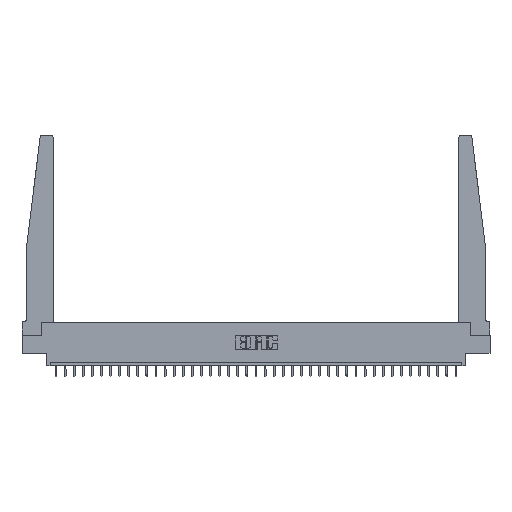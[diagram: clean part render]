
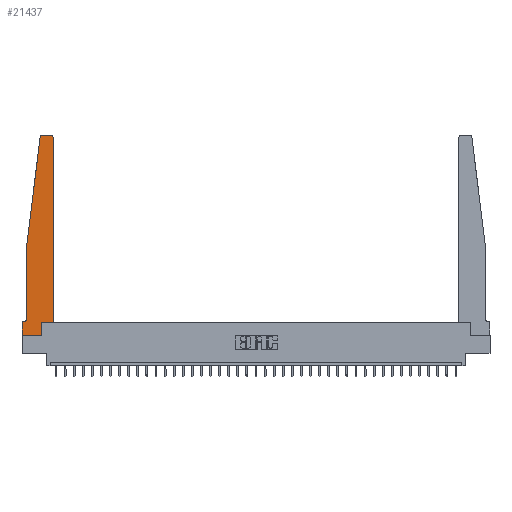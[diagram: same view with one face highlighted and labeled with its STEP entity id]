
A CAD part, top view. The second image highlights one B-rep face of the part: STEP entity #21437.
In plain terms, the highlighted planar face has unit normal (0, 0, 1).
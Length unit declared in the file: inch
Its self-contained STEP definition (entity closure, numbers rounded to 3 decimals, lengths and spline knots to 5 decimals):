
#78 = CARTESIAN_POINT ( 'NONE',  ( 0.015, 0.2375, 0.37 ) ) ;
#436 = CARTESIAN_POINT ( 'NONE',  ( 0., 0., 0.37 ) ) ;
#1081 = ORIENTED_EDGE ( 'NONE', *, *, #4601, .T. ) ;
#1486 = DIRECTION ( 'NONE',  ( 0., -1., 0. ) ) ;
#1632 = CARTESIAN_POINT ( 'NONE',  ( 0., 0., 0.37 ) ) ;
#1698 = CARTESIAN_POINT ( 'NONE',  ( 0.2605, 0., 0.37 ) ) ;
#1719 = VECTOR ( 'NONE', #17301, 39.37008 ) ;
#1844 = CARTESIAN_POINT ( 'NONE',  ( 0.425, 0.18, 0.37 ) ) ;
#1995 = EDGE_CURVE ( 'NONE', #14347, #32443, #30287, .T. ) ;
#2155 = CARTESIAN_POINT ( 'NONE',  ( 0., 0., 0.37 ) ) ;
#2578 = DIRECTION ( 'NONE',  ( 1., 0., 0. ) ) ;
#2686 = EDGE_LOOP ( 'NONE', ( #14215, #1081, #5390, #25383, #31461, #9078, #31612, #27559, #22844, #9405, #11229, #5783 ) ) ;
#2786 = EDGE_CURVE ( 'NONE', #32053, #6396, #11016, .T. ) ;
#2797 = VERTEX_POINT ( 'NONE', #1698 ) ;
#3296 = VERTEX_POINT ( 'NONE', #436 ) ;
#4121 = EDGE_CURVE ( 'NONE', #10559, #21820, #5808, .T. ) ;
#4601 = EDGE_CURVE ( 'NONE', #23123, #32053, #27783, .T. ) ;
#4746 = CARTESIAN_POINT ( 'NONE',  ( 0.425, 0.18, 0.37 ) ) ;
#5390 = ORIENTED_EDGE ( 'NONE', *, *, #2786, .T. ) ;
#5399 = DIRECTION ( 'NONE',  ( 0., 0., 1. ) ) ;
#5516 = CIRCLE ( 'NONE', #15982, 0.05 ) ;
#5783 = ORIENTED_EDGE ( 'NONE', *, *, #4121, .T. ) ;
#5808 = CIRCLE ( 'NONE', #29181, 0.03 ) ;
#6149 = CARTESIAN_POINT ( 'NONE',  ( 0.2605, 0.18, 0.37 ) ) ;
#6396 = VERTEX_POINT ( 'NONE', #20817 ) ;
#6866 = DIRECTION ( 'NONE',  ( 0., -1., 0. ) ) ;
#7437 = EDGE_CURVE ( 'NONE', #2797, #14347, #8352, .T. ) ;
#7590 = DIRECTION ( 'NONE',  ( 1., 0., 0. ) ) ;
#7659 = VERTEX_POINT ( 'NONE', #28239 ) ;
#7867 = EDGE_CURVE ( 'NONE', #32443, #10559, #13844, .T. ) ;
#8148 = CARTESIAN_POINT ( 'NONE',  ( 0.425, 2.72, 0.37 ) ) ;
#8352 = LINE ( 'NONE', #6149, #1719 ) ;
#8532 = EDGE_CURVE ( 'NONE', #21820, #23123, #30784, .T. ) ;
#8833 = VECTOR ( 'NONE', #8940, 39.37008 ) ;
#8940 = DIRECTION ( 'NONE',  ( -1., 0., 0. ) ) ;
#9078 = ORIENTED_EDGE ( 'NONE', *, *, #15587, .T. ) ;
#9405 = ORIENTED_EDGE ( 'NONE', *, *, #1995, .T. ) ;
#10381 = DIRECTION ( 'NONE',  ( 1., 0., 0. ) ) ;
#10559 = VERTEX_POINT ( 'NONE', #8148 ) ;
#10767 = VECTOR ( 'NONE', #26621, 39.37008 ) ;
#11016 = LINE ( 'NONE', #21911, #14957 ) ;
#11229 = ORIENTED_EDGE ( 'NONE', *, *, #7867, .T. ) ;
#11241 = DIRECTION ( 'NONE',  ( 1., 0., 0. ) ) ;
#11785 = DIRECTION ( 'NONE',  ( 0., 1., 0. ) ) ;
#12787 = PLANE ( 'NONE',  #24718 ) ;
#12901 = DIRECTION ( 'NONE',  ( 0., 0., 1. ) ) ;
#13844 = LINE ( 'NONE', #4746, #32254 ) ;
#14215 = ORIENTED_EDGE ( 'NONE', *, *, #8532, .T. ) ;
#14238 = DIRECTION ( 'NONE',  ( 1., 0., 0. ) ) ;
#14347 = VERTEX_POINT ( 'NONE', #21317 ) ;
#14620 = DIRECTION ( 'NONE',  ( -0.122, -0.992, 0. ) ) ;
#14957 = VECTOR ( 'NONE', #14620, 39.37008 ) ;
#15138 = CARTESIAN_POINT ( 'NONE',  ( 0.27653, 2.75, 0.37 ) ) ;
#15587 = EDGE_CURVE ( 'NONE', #7659, #31691, #28891, .T. ) ;
#15982 = AXIS2_PLACEMENT_3D ( 'NONE', #78, #24930, #17506 ) ;
#16224 = CARTESIAN_POINT ( 'NONE',  ( 0.395, 2.72, 0.37 ) ) ;
#16771 = CARTESIAN_POINT ( 'NONE',  ( 0.065, 1.25, 0.37 ) ) ;
#17044 = CARTESIAN_POINT ( 'NONE',  ( 0.065, 0.2375, 0.37 ) ) ;
#17201 = CARTESIAN_POINT ( 'NONE',  ( 0.24675, 2.72367, 0.37 ) ) ;
#17301 = DIRECTION ( 'NONE',  ( 0., 1., 0. ) ) ;
#17506 = DIRECTION ( 'NONE',  ( -1., 0., 0. ) ) ;
#19247 = LINE ( 'NONE', #2155, #21205 ) ;
#19880 = VERTEX_POINT ( 'NONE', #17044 ) ;
#20494 = CARTESIAN_POINT ( 'NONE',  ( 0.27653, 2.72, 0.37 ) ) ;
#20817 = CARTESIAN_POINT ( 'NONE',  ( 0.065, 1.25, 0.37 ) ) ;
#21205 = VECTOR ( 'NONE', #2578, 39.37008 ) ;
#21317 = CARTESIAN_POINT ( 'NONE',  ( 0.2605, 0.18, 0.37 ) ) ;
#21415 = CARTESIAN_POINT ( 'NONE',  ( 0.065, 0.1875, 0.37 ) ) ;
#21437 = ADVANCED_FACE ( 'NONE', ( #24043 ), #12787, .T. ) ;
#21820 = VERTEX_POINT ( 'NONE', #31414 ) ;
#21911 = CARTESIAN_POINT ( 'NONE',  ( 0.065, 1.25, 0.37 ) ) ;
#22844 = ORIENTED_EDGE ( 'NONE', *, *, #7437, .T. ) ;
#23088 = LINE ( 'NONE', #1632, #30123 ) ;
#23123 = VERTEX_POINT ( 'NONE', #15138 ) ;
#23212 = EDGE_CURVE ( 'NONE', #19880, #7659, #5516, .T. ) ;
#23755 = DIRECTION ( 'NONE',  ( 0., 0., 1. ) ) ;
#24043 = FACE_OUTER_BOUND ( 'NONE', #2686, .T. ) ;
#24074 = CARTESIAN_POINT ( 'NONE',  ( 0.425, 0.18, 0.37 ) ) ;
#24140 = CARTESIAN_POINT ( 'NONE',  ( 0.25, 2.75, 0.37 ) ) ;
#24223 = VECTOR ( 'NONE', #1486, 39.37008 ) ;
#24374 = EDGE_CURVE ( 'NONE', #3296, #2797, #19247, .T. ) ;
#24579 = LINE ( 'NONE', #16771, #24223 ) ;
#24718 = AXIS2_PLACEMENT_3D ( 'NONE', #27707, #12901, #10381 ) ;
#24930 = DIRECTION ( 'NONE',  ( 0., 0., -1. ) ) ;
#24989 = CARTESIAN_POINT ( 'NONE',  ( 0., 0.1875, 0.37 ) ) ;
#25383 = ORIENTED_EDGE ( 'NONE', *, *, #29550, .T. ) ;
#25432 = AXIS2_PLACEMENT_3D ( 'NONE', #20494, #5399, #7590 ) ;
#26621 = DIRECTION ( 'NONE',  ( -1., 0., 0. ) ) ;
#27559 = ORIENTED_EDGE ( 'NONE', *, *, #24374, .T. ) ;
#27707 = CARTESIAN_POINT ( 'NONE',  ( 0., 0.1875, 0.37 ) ) ;
#27783 = CIRCLE ( 'NONE', #25432, 0.03 ) ;
#27932 = VECTOR ( 'NONE', #14238, 39.37008 ) ;
#28239 = CARTESIAN_POINT ( 'NONE',  ( 0.015, 0.1875, 0.37 ) ) ;
#28240 = EDGE_CURVE ( 'NONE', #31691, #3296, #23088, .T. ) ;
#28891 = LINE ( 'NONE', #21415, #8833 ) ;
#29181 = AXIS2_PLACEMENT_3D ( 'NONE', #16224, #23755, #11241 ) ;
#29550 = EDGE_CURVE ( 'NONE', #6396, #19880, #24579, .T. ) ;
#30123 = VECTOR ( 'NONE', #6866, 39.37008 ) ;
#30287 = LINE ( 'NONE', #1844, #27932 ) ;
#30784 = LINE ( 'NONE', #24140, #10767 ) ;
#31414 = CARTESIAN_POINT ( 'NONE',  ( 0.395, 2.75, 0.37 ) ) ;
#31461 = ORIENTED_EDGE ( 'NONE', *, *, #23212, .T. ) ;
#31612 = ORIENTED_EDGE ( 'NONE', *, *, #28240, .T. ) ;
#31691 = VERTEX_POINT ( 'NONE', #24989 ) ;
#32053 = VERTEX_POINT ( 'NONE', #17201 ) ;
#32254 = VECTOR ( 'NONE', #11785, 39.37008 ) ;
#32443 = VERTEX_POINT ( 'NONE', #24074 ) ;
